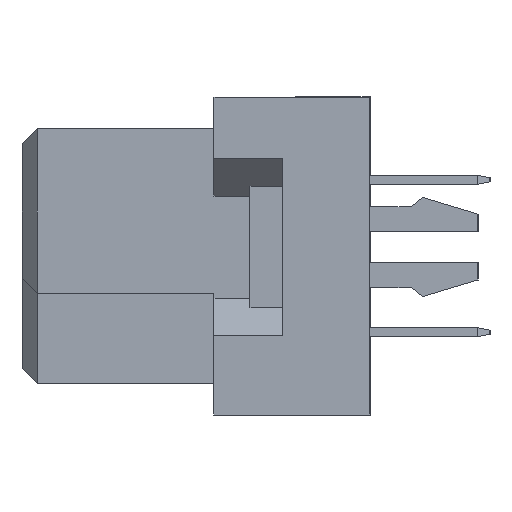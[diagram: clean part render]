
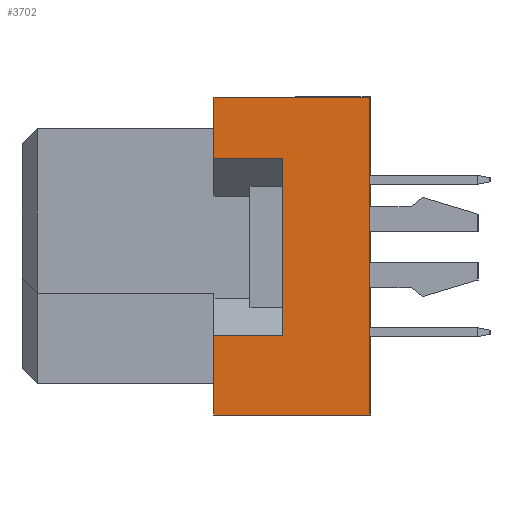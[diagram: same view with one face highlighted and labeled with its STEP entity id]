
A CAD part, left-side view. The second image highlights one B-rep face of the part: STEP entity #3702.
In plain terms, the highlighted planar face has unit normal (-1, 0, 0).
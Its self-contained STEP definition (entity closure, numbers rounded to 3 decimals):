
#72 = EDGE_CURVE ( 'NONE', #25392, #5068, #25653, .T. ) ;
#1261 = CARTESIAN_POINT ( 'NONE',  ( -47.5, -8.7, -2.65 ) ) ;
#1803 = EDGE_CURVE ( 'NONE', #20610, #7575, #5245, .T. ) ;
#3006 = LINE ( 'NONE', #21448, #20133 ) ;
#3702 = ADVANCED_FACE ( 'NONE', ( #31405 ), #33698, .T. ) ;
#4062 = ORIENTED_EDGE ( 'NONE', *, *, #39875, .F. ) ;
#5026 = VECTOR ( 'NONE', #8919, 1000. ) ;
#5068 = VERTEX_POINT ( 'NONE', #16375 ) ;
#5245 = LINE ( 'NONE', #7920, #8734 ) ;
#7017 = DIRECTION ( 'NONE',  ( 0., 0., 1. ) ) ;
#7575 = VERTEX_POINT ( 'NONE', #25864 ) ;
#7920 = CARTESIAN_POINT ( 'NONE',  ( -47.5, -6.4, -5.3 ) ) ;
#8032 = VERTEX_POINT ( 'NONE', #12918 ) ;
#8540 = VECTOR ( 'NONE', #31458, 1000. ) ;
#8734 = VECTOR ( 'NONE', #17747, 1000. ) ;
#8919 = DIRECTION ( 'NONE',  ( 0., 0., 1. ) ) ;
#9123 = ORIENTED_EDGE ( 'NONE', *, *, #27087, .T. ) ;
#10159 = LINE ( 'NONE', #12814, #8540 ) ;
#11682 = CARTESIAN_POINT ( 'NONE',  ( -47.5, -11.6, 5.3 ) ) ;
#12180 = DIRECTION ( 'NONE',  ( 0., 0., 1. ) ) ;
#12781 = CARTESIAN_POINT ( 'NONE',  ( -47.5, -6.4, 3.25 ) ) ;
#12814 = CARTESIAN_POINT ( 'NONE',  ( -47.5, -8.7, -2.65 ) ) ;
#12889 = VECTOR ( 'NONE', #24156, 1000. ) ;
#12918 = CARTESIAN_POINT ( 'NONE',  ( -47.5, -11.6, -5.3 ) ) ;
#12998 = ORIENTED_EDGE ( 'NONE', *, *, #20367, .F. ) ;
#13246 = LINE ( 'NONE', #19994, #26021 ) ;
#13587 = LINE ( 'NONE', #20138, #38952 ) ;
#14638 = VERTEX_POINT ( 'NONE', #38935 ) ;
#16375 = CARTESIAN_POINT ( 'NONE',  ( -47.5, -8.7, 3.25 ) ) ;
#16854 = VERTEX_POINT ( 'NONE', #26081 ) ;
#17747 = DIRECTION ( 'NONE',  ( 0., 0., 1. ) ) ;
#18028 = LINE ( 'NONE', #11682, #12889 ) ;
#18573 = DIRECTION ( 'NONE',  ( 0., 0., 1. ) ) ;
#19447 = EDGE_CURVE ( 'NONE', #8032, #14638, #37554, .T. ) ;
#19994 = CARTESIAN_POINT ( 'NONE',  ( -47.5, -11.6, -5.3 ) ) ;
#20133 = VECTOR ( 'NONE', #18573, 1000. ) ;
#20138 = CARTESIAN_POINT ( 'NONE',  ( -47.5, -8.7, 3.25 ) ) ;
#20367 = EDGE_CURVE ( 'NONE', #8032, #27638, #13246, .T. ) ;
#20610 = VERTEX_POINT ( 'NONE', #12781 ) ;
#21264 = EDGE_CURVE ( 'NONE', #14638, #7575, #18028, .T. ) ;
#21448 = CARTESIAN_POINT ( 'NONE',  ( -47.5, -6.4, -5.3 ) ) ;
#21794 = DIRECTION ( 'NONE',  ( -1., 0., 0. ) ) ;
#22488 = CARTESIAN_POINT ( 'NONE',  ( -47.5, -8.7, -2.65 ) ) ;
#24156 = DIRECTION ( 'NONE',  ( 0., 1., 0. ) ) ;
#24252 = CARTESIAN_POINT ( 'NONE',  ( -47.5, -11.6, 5.3 ) ) ;
#25392 = VERTEX_POINT ( 'NONE', #22488 ) ;
#25653 = LINE ( 'NONE', #1261, #26541 ) ;
#25864 = CARTESIAN_POINT ( 'NONE',  ( -47.5, -6.4, 5.3 ) ) ;
#26021 = VECTOR ( 'NONE', #29403, 1000. ) ;
#26081 = CARTESIAN_POINT ( 'NONE',  ( -47.5, -6.4, -2.65 ) ) ;
#26173 = ORIENTED_EDGE ( 'NONE', *, *, #1803, .F. ) ;
#26541 = VECTOR ( 'NONE', #7017, 1000. ) ;
#27087 = EDGE_CURVE ( 'NONE', #25392, #16854, #10159, .T. ) ;
#27638 = VERTEX_POINT ( 'NONE', #36462 ) ;
#28595 = ORIENTED_EDGE ( 'NONE', *, *, #19447, .T. ) ;
#28884 = AXIS2_PLACEMENT_3D ( 'NONE', #24252, #21794, #12180 ) ;
#29403 = DIRECTION ( 'NONE',  ( 0., 1., 0. ) ) ;
#31405 = FACE_OUTER_BOUND ( 'NONE', #36506, .T. ) ;
#31458 = DIRECTION ( 'NONE',  ( 0., 1., 0. ) ) ;
#33698 = PLANE ( 'NONE',  #28884 ) ;
#34031 = ORIENTED_EDGE ( 'NONE', *, *, #35436, .F. ) ;
#35436 = EDGE_CURVE ( 'NONE', #5068, #20610, #13587, .T. ) ;
#36462 = CARTESIAN_POINT ( 'NONE',  ( -47.5, -6.4, -5.3 ) ) ;
#36506 = EDGE_LOOP ( 'NONE', ( #9123, #4062, #12998, #28595, #37112, #26173, #34031, #36785 ) ) ;
#36785 = ORIENTED_EDGE ( 'NONE', *, *, #72, .F. ) ;
#36965 = CARTESIAN_POINT ( 'NONE',  ( -47.5, -11.6, 5.3 ) ) ;
#37112 = ORIENTED_EDGE ( 'NONE', *, *, #21264, .T. ) ;
#37554 = LINE ( 'NONE', #36965, #5026 ) ;
#38935 = CARTESIAN_POINT ( 'NONE',  ( -47.5, -11.6, 5.3 ) ) ;
#38952 = VECTOR ( 'NONE', #39168, 1000. ) ;
#39168 = DIRECTION ( 'NONE',  ( 0., 1., 0. ) ) ;
#39875 = EDGE_CURVE ( 'NONE', #27638, #16854, #3006, .T. ) ;
